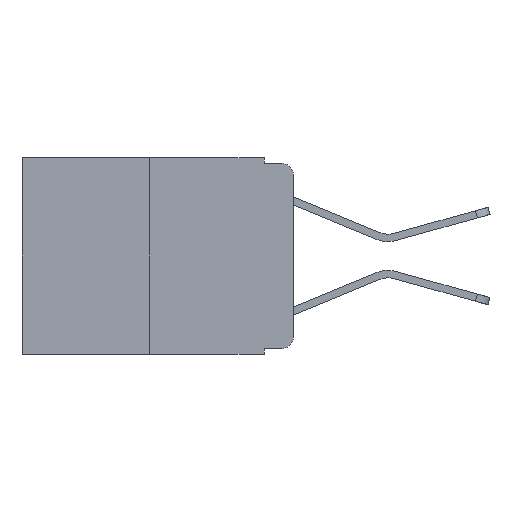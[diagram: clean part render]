
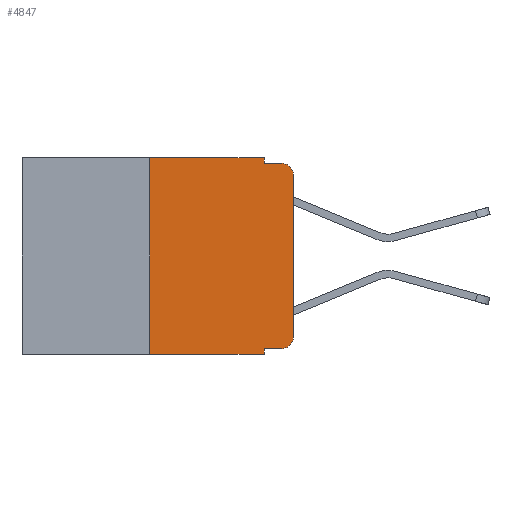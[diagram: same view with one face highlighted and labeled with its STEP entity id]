
A CAD part, left-side view. The second image highlights one B-rep face of the part: STEP entity #4847.
In plain terms, the highlighted planar face has unit normal (-1, 0, 0).
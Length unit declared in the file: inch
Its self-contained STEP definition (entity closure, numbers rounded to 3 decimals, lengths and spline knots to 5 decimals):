
#316 = CARTESIAN_POINT ( 'NONE',  ( 0., 0.051, 0. ) ) ;
#337 = DIRECTION ( 'NONE',  ( 0., 0., -1. ) ) ;
#538 = VERTEX_POINT ( 'NONE', #1564 ) ;
#663 = ORIENTED_EDGE ( 'NONE', *, *, #10434, .F. ) ;
#671 = CARTESIAN_POINT ( 'NONE',  ( 0., 0., -0.313 ) ) ;
#876 = DIRECTION ( 'NONE',  ( -1., 0., 0. ) ) ;
#1063 = CARTESIAN_POINT ( 'NONE',  ( 0., 0.051, -0.333 ) ) ;
#1418 = EDGE_CURVE ( 'NONE', #11697, #2714, #6656, .T. ) ;
#1475 = CARTESIAN_POINT ( 'NONE',  ( 0., 0.051, -0.01 ) ) ;
#1488 = VERTEX_POINT ( 'NONE', #7803 ) ;
#1564 = CARTESIAN_POINT ( 'NONE',  ( 0., 0.051, -0.333 ) ) ;
#1667 = DIRECTION ( 'NONE',  ( 0., 0., -1. ) ) ;
#1728 = EDGE_CURVE ( 'NONE', #538, #9575, #5663, .T. ) ;
#1776 = DIRECTION ( 'NONE',  ( 0., 0., -1. ) ) ;
#1832 = CARTESIAN_POINT ( 'NONE',  ( 0., 0.25, -0.343 ) ) ;
#1958 = EDGE_CURVE ( 'NONE', #4583, #6542, #5802, .T. ) ;
#2150 = DIRECTION ( 'NONE',  ( 0., -1., 0. ) ) ;
#2188 = ORIENTED_EDGE ( 'NONE', *, *, #2368, .T. ) ;
#2271 = CARTESIAN_POINT ( 'NONE',  ( 0., 0.473, 0. ) ) ;
#2368 = EDGE_CURVE ( 'NONE', #9575, #4583, #10864, .T. ) ;
#2391 = PLANE ( 'NONE',  #4084 ) ;
#2714 = VERTEX_POINT ( 'NONE', #10441 ) ;
#2891 = DIRECTION ( 'NONE',  ( 0., 0., -1. ) ) ;
#2905 = VECTOR ( 'NONE', #2150, 39.37008 ) ;
#3051 = CARTESIAN_POINT ( 'NONE',  ( 0., 0.02, -0.313 ) ) ;
#3075 = VECTOR ( 'NONE', #8201, 39.37008 ) ;
#3237 = ORIENTED_EDGE ( 'NONE', *, *, #4225, .F. ) ;
#3390 = LINE ( 'NONE', #9104, #5834 ) ;
#3410 = VERTEX_POINT ( 'NONE', #316 ) ;
#3831 = ORIENTED_EDGE ( 'NONE', *, *, #1418, .T. ) ;
#4084 = AXIS2_PLACEMENT_3D ( 'NONE', #2271, #6477, #337 ) ;
#4200 = AXIS2_PLACEMENT_3D ( 'NONE', #6475, #876, #7385 ) ;
#4209 = FACE_OUTER_BOUND ( 'NONE', #11569, .T. ) ;
#4225 = EDGE_CURVE ( 'NONE', #9961, #3410, #5526, .T. ) ;
#4228 = VECTOR ( 'NONE', #7922, 39.37008 ) ;
#4388 = ORIENTED_EDGE ( 'NONE', *, *, #1728, .T. ) ;
#4583 = VERTEX_POINT ( 'NONE', #671 ) ;
#4605 = CARTESIAN_POINT ( 'NONE',  ( 0., 0.473, 0. ) ) ;
#4847 = ADVANCED_FACE ( 'NONE', ( #4209 ), #2391, .F. ) ;
#5023 = LINE ( 'NONE', #1475, #9489 ) ;
#5228 = CARTESIAN_POINT ( 'NONE',  ( 0., 0., 0. ) ) ;
#5392 = ORIENTED_EDGE ( 'NONE', *, *, #8150, .F. ) ;
#5405 = CARTESIAN_POINT ( 'NONE',  ( 0., 0.02, -0.01 ) ) ;
#5507 = VECTOR ( 'NONE', #8868, 39.37008 ) ;
#5526 = LINE ( 'NONE', #4605, #3075 ) ;
#5663 = LINE ( 'NONE', #1063, #2905 ) ;
#5802 = LINE ( 'NONE', #5228, #5507 ) ;
#5834 = VECTOR ( 'NONE', #7298, 39.37008 ) ;
#5981 = ORIENTED_EDGE ( 'NONE', *, *, #9875, .F. ) ;
#6269 = VECTOR ( 'NONE', #1667, 39.37008 ) ;
#6322 = EDGE_CURVE ( 'NONE', #6542, #8694, #10696, .T. ) ;
#6475 = CARTESIAN_POINT ( 'NONE',  ( 0., 0.02, -0.03 ) ) ;
#6477 = DIRECTION ( 'NONE',  ( 1., 0., 0. ) ) ;
#6542 = VERTEX_POINT ( 'NONE', #8548 ) ;
#6656 = LINE ( 'NONE', #9021, #4228 ) ;
#7245 = ORIENTED_EDGE ( 'NONE', *, *, #1958, .T. ) ;
#7298 = DIRECTION ( 'NONE',  ( 0., 0., 1. ) ) ;
#7315 = CARTESIAN_POINT ( 'NONE',  ( 0., 0.051, 0. ) ) ;
#7338 = AXIS2_PLACEMENT_3D ( 'NONE', #3051, #8689, #2891 ) ;
#7385 = DIRECTION ( 'NONE',  ( 0., 0., -1. ) ) ;
#7803 = CARTESIAN_POINT ( 'NONE',  ( 0., 0.051, -0.01 ) ) ;
#7922 = DIRECTION ( 'NONE',  ( 0., -1., 0. ) ) ;
#8150 = EDGE_CURVE ( 'NONE', #1488, #8694, #5023, .T. ) ;
#8201 = DIRECTION ( 'NONE',  ( 0., -1., 0. ) ) ;
#8548 = CARTESIAN_POINT ( 'NONE',  ( 0., 0., -0.03 ) ) ;
#8676 = ORIENTED_EDGE ( 'NONE', *, *, #11550, .F. ) ;
#8684 = LINE ( 'NONE', #11489, #6269 ) ;
#8689 = DIRECTION ( 'NONE',  ( -1., 0., 0. ) ) ;
#8694 = VERTEX_POINT ( 'NONE', #5405 ) ;
#8825 = LINE ( 'NONE', #7315, #9087 ) ;
#8852 = DIRECTION ( 'NONE',  ( 0., -1., 0. ) ) ;
#8868 = DIRECTION ( 'NONE',  ( 0., 0., 1. ) ) ;
#9021 = CARTESIAN_POINT ( 'NONE',  ( 0., 0.473, -0.343 ) ) ;
#9087 = VECTOR ( 'NONE', #1776, 39.37008 ) ;
#9104 = CARTESIAN_POINT ( 'NONE',  ( 0., 0.25, 0. ) ) ;
#9340 = CARTESIAN_POINT ( 'NONE',  ( 0., 0.25, 0. ) ) ;
#9489 = VECTOR ( 'NONE', #8852, 39.37008 ) ;
#9493 = CARTESIAN_POINT ( 'NONE',  ( 0., 0.02, -0.333 ) ) ;
#9575 = VERTEX_POINT ( 'NONE', #9493 ) ;
#9850 = ORIENTED_EDGE ( 'NONE', *, *, #6322, .T. ) ;
#9875 = EDGE_CURVE ( 'NONE', #11697, #9961, #3390, .T. ) ;
#9961 = VERTEX_POINT ( 'NONE', #9340 ) ;
#10434 = EDGE_CURVE ( 'NONE', #3410, #1488, #8825, .T. ) ;
#10441 = CARTESIAN_POINT ( 'NONE',  ( 0., 0.051, -0.343 ) ) ;
#10696 = CIRCLE ( 'NONE', #4200, 0.02 ) ;
#10864 = CIRCLE ( 'NONE', #7338, 0.02 ) ;
#11489 = CARTESIAN_POINT ( 'NONE',  ( 0., 0.051, 0. ) ) ;
#11550 = EDGE_CURVE ( 'NONE', #538, #2714, #8684, .T. ) ;
#11569 = EDGE_LOOP ( 'NONE', ( #7245, #9850, #5392, #663, #3237, #5981, #3831, #8676, #4388, #2188 ) ) ;
#11697 = VERTEX_POINT ( 'NONE', #1832 ) ;
